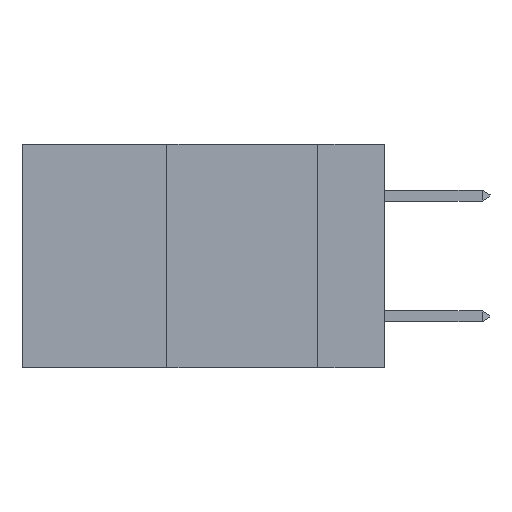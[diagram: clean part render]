
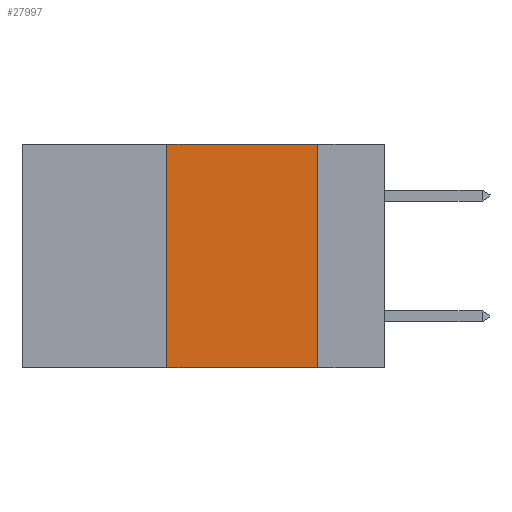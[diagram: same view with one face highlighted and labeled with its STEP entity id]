
A CAD part, left-side view. The second image highlights one B-rep face of the part: STEP entity #27997.
In plain terms, the highlighted planar face has unit normal (-1, 0, 0).
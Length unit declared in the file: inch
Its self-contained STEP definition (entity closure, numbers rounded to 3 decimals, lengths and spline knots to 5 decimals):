
#138 = ORIENTED_EDGE ( 'NONE', *, *, #2816, .F. ) ;
#2172 = CARTESIAN_POINT ( 'NONE',  ( 0., 0.36, 0. ) ) ;
#2598 = LINE ( 'NONE', #11198, #29536 ) ;
#2816 = EDGE_CURVE ( 'NONE', #24075, #17963, #2598, .T. ) ;
#3112 = LINE ( 'NONE', #2172, #20704 ) ;
#4117 = EDGE_LOOP ( 'NONE', ( #138, #23666, #11930, #31301 ) ) ;
#5118 = CARTESIAN_POINT ( 'NONE',  ( 0., 0.11, 0. ) ) ;
#6672 = VECTOR ( 'NONE', #17416, 39.37008 ) ;
#7150 = DIRECTION ( 'NONE',  ( 0., 0., -1. ) ) ;
#11198 = CARTESIAN_POINT ( 'NONE',  ( 0., 0.11, 0. ) ) ;
#11930 = ORIENTED_EDGE ( 'NONE', *, *, #32713, .F. ) ;
#12757 = DIRECTION ( 'NONE',  ( 1., 0., 0. ) ) ;
#13609 = LINE ( 'NONE', #29872, #6672 ) ;
#15396 = DIRECTION ( 'NONE',  ( 0., 0., 1. ) ) ;
#15501 = CARTESIAN_POINT ( 'NONE',  ( 0., 0.6, -0.37 ) ) ;
#15618 = CARTESIAN_POINT ( 'NONE',  ( 0., 0.11, -0.37 ) ) ;
#17416 = DIRECTION ( 'NONE',  ( 0., -1., 0. ) ) ;
#17963 = VERTEX_POINT ( 'NONE', #15618 ) ;
#19480 = VECTOR ( 'NONE', #31509, 39.37008 ) ;
#20704 = VECTOR ( 'NONE', #15396, 39.37008 ) ;
#20755 = CARTESIAN_POINT ( 'NONE',  ( 0., 0.36, 0. ) ) ;
#21448 = FACE_OUTER_BOUND ( 'NONE', #4117, .T. ) ;
#23044 = PLANE ( 'NONE',  #28516 ) ;
#23666 = ORIENTED_EDGE ( 'NONE', *, *, #28479, .F. ) ;
#24075 = VERTEX_POINT ( 'NONE', #5118 ) ;
#25623 = LINE ( 'NONE', #15501, #19480 ) ;
#27997 = ADVANCED_FACE ( 'NONE', ( #21448 ), #23044, .F. ) ;
#28132 = VERTEX_POINT ( 'NONE', #20755 ) ;
#28479 = EDGE_CURVE ( 'NONE', #28132, #24075, #13609, .T. ) ;
#28516 = AXIS2_PLACEMENT_3D ( 'NONE', #30923, #12757, #7150 ) ;
#29536 = VECTOR ( 'NONE', #32205, 39.37008 ) ;
#29872 = CARTESIAN_POINT ( 'NONE',  ( 0., 0.6, 0. ) ) ;
#30923 = CARTESIAN_POINT ( 'NONE',  ( 0., 0.6, 0. ) ) ;
#31301 = ORIENTED_EDGE ( 'NONE', *, *, #32734, .T. ) ;
#31509 = DIRECTION ( 'NONE',  ( 0., -1., 0. ) ) ;
#32205 = DIRECTION ( 'NONE',  ( 0., 0., -1. ) ) ;
#32302 = CARTESIAN_POINT ( 'NONE',  ( 0., 0.36, -0.37 ) ) ;
#32357 = VERTEX_POINT ( 'NONE', #32302 ) ;
#32713 = EDGE_CURVE ( 'NONE', #32357, #28132, #3112, .T. ) ;
#32734 = EDGE_CURVE ( 'NONE', #32357, #17963, #25623, .T. ) ;
